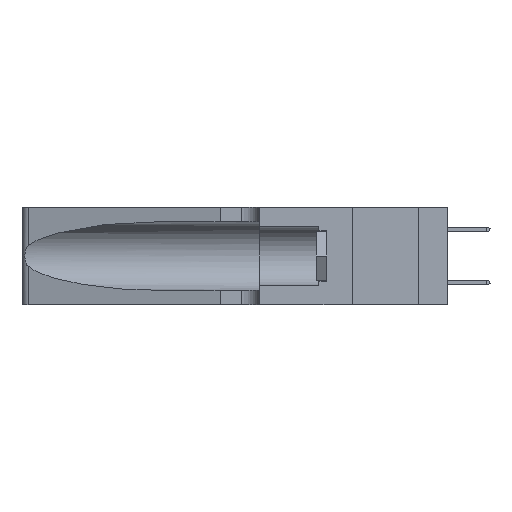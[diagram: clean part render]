
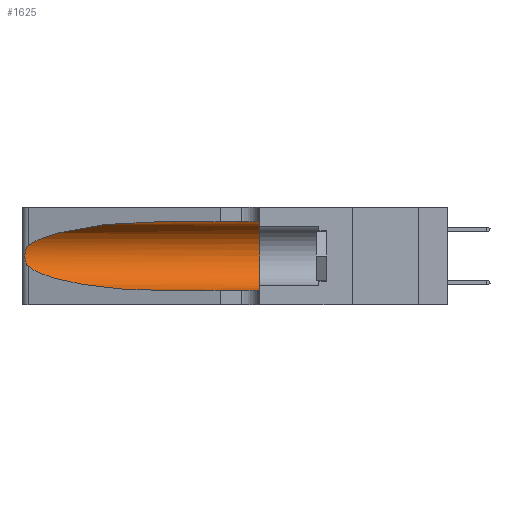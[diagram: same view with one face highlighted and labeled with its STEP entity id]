
A CAD part, left-side view. The second image highlights one B-rep face of the part: STEP entity #1625.
In plain terms, the highlighted cylindrical face has radius 3.308 mm (diameter 6.617 mm), a partial arc.
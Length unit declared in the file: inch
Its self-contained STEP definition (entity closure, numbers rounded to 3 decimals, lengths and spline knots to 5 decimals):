
#87 = VERTEX_POINT ( 'NONE', #21972 ) ;
#1451 = EDGE_CURVE ( 'NONE', #5582, #16488, #2041, .T. ) ;
#1625 = ADVANCED_FACE ( 'NONE', ( #29421 ), #23085, .F. ) ;
#2041 = B_SPLINE_CURVE_WITH_KNOTS ( 'NONE', 3,
 ( #26276, #11181, #11412, #3783, #18534, #28564, #6456, #8677, #25912, #31040, #31164, #11291, #13688, #6216 ),
 .UNSPECIFIED., .F., .F.,
 ( 4, 2, 2, 2, 2, 2, 4 ),
 ( 0., 0.00027, 0.00053, 0.00107, 0.0016, 0.00187, 0.00214 ),
 .UNSPECIFIED. ) ;
#3321 = CARTESIAN_POINT ( 'NONE',  ( 0.1305, 0.35, 0.185 ) ) ;
#3783 = CARTESIAN_POINT ( 'NONE',  ( 0.25787, 1.23484, 0.2124 ) ) ;
#3870 = DIRECTION ( 'NONE',  ( 0., -1., 0. ) ) ;
#4662 = ORIENTED_EDGE ( 'NONE', *, *, #28804, .T. ) ;
#5500 = DIRECTION ( 'NONE',  ( 0., -1., 0. ) ) ;
#5582 = VERTEX_POINT ( 'NONE', #7429 ) ;
#5670 = CARTESIAN_POINT ( 'NONE',  ( 0.25487, 1.22718, 0.14631 ) ) ;
#6216 = CARTESIAN_POINT ( 'NONE',  ( 0.25487, 1.22718, 0.14631 ) ) ;
#6456 = CARTESIAN_POINT ( 'NONE',  ( 0.26075, 1.23896, 0.19203 ) ) ;
#6742 = VERTEX_POINT ( 'NONE', #17976 ) ;
#7429 = CARTESIAN_POINT ( 'NONE',  ( 0.25487, 1.22718, 0.22369 ) ) ;
#7825 = CARTESIAN_POINT ( 'NONE',  ( 0.25487, 1.22718, 0.14631 ) ) ;
#8677 = CARTESIAN_POINT ( 'NONE',  ( 0.26075, 1.23896, 0.178 ) ) ;
#9028 = CARTESIAN_POINT ( 'NONE',  ( 0.18966, 0.96281, 0.05475 ) ) ;
#9557 = ORIENTED_EDGE ( 'NONE', *, *, #1451, .T. ) ;
#9734 = CARTESIAN_POINT ( 'NONE',  ( 0.18966, 0.96281, 0.31525 ) ) ;
#10636 = VERTEX_POINT ( 'NONE', #16142 ) ;
#10696 = DIRECTION ( 'NONE',  ( 0., 1., 0. ) ) ;
#11151 = CARTESIAN_POINT ( 'NONE',  ( 0.1305, 1.61858, 0.05475 ) ) ;
#11181 = CARTESIAN_POINT ( 'NONE',  ( 0.25555, 1.22994, 0.2215 ) ) ;
#11276 = EDGE_CURVE ( 'NONE', #29464, #10636, #20356, .T. ) ;
#11291 = CARTESIAN_POINT ( 'NONE',  ( 0.25639, 1.23186, 0.15144 ) ) ;
#11412 = CARTESIAN_POINT ( 'NONE',  ( 0.25639, 1.23184, 0.21858 ) ) ;
#11788 = ORIENTED_EDGE ( 'NONE', *, *, #14087, .F. ) ;
#13055 = CARTESIAN_POINT ( 'NONE',  ( 0.1305, 1.61858, 0.31525 ) ) ;
#13688 = CARTESIAN_POINT ( 'NONE',  ( 0.25555, 1.22993, 0.14849 ) ) ;
#14087 = EDGE_CURVE ( 'NONE', #10636, #87, #26049, .T. ) ;
#14395 = CARTESIAN_POINT ( 'NONE',  ( 0.2373, 1.15595, 0.28018 ) ) ;
#14895 = ORIENTED_EDGE ( 'NONE', *, *, #11276, .F. ) ;
#15634 = AXIS2_PLACEMENT_3D ( 'NONE', #3321, #10696, #30573 ) ;
#16142 = CARTESIAN_POINT ( 'NONE',  ( 0.1305, 0.35, 0.31525 ) ) ;
#16488 = VERTEX_POINT ( 'NONE', #7825 ) ;
#16965 =( BOUNDED_CURVE ( )  B_SPLINE_CURVE ( 3, ( #17009, #9734, #14395, #19265 ),
 .UNSPECIFIED., .F., .T. ) 
 B_SPLINE_CURVE_WITH_KNOTS ( ( 4, 4 ),
 ( 1.5708, 2.84003 ),
 .UNSPECIFIED. ) 
 CURVE ( )  GEOMETRIC_REPRESENTATION_ITEM ( )  RATIONAL_B_SPLINE_CURVE ( ( 1., 0.87, 0.87, 1. ) ) 
 REPRESENTATION_ITEM ( '' )  );
#17009 = CARTESIAN_POINT ( 'NONE',  ( 0.1305, 0.72297, 0.31525 ) ) ;
#17976 = CARTESIAN_POINT ( 'NONE',  ( 0.1305, 0.72297, 0.05475 ) ) ;
#18033 = VECTOR ( 'NONE', #5500, 39.37008 ) ;
#18534 = CARTESIAN_POINT ( 'NONE',  ( 0.25854, 1.2359, 0.20912 ) ) ;
#18593 = VECTOR ( 'NONE', #3870, 39.37008 ) ;
#19202 = DIRECTION ( 'NONE',  ( 0., 0., -1. ) ) ;
#19265 = CARTESIAN_POINT ( 'NONE',  ( 0.25487, 1.22718, 0.22369 ) ) ;
#19384 = LINE ( 'NONE', #11151, #18593 ) ;
#20272 =( BOUNDED_CURVE ( )  B_SPLINE_CURVE ( 3, ( #5670, #22969, #9028, #26531 ),
 .UNSPECIFIED., .F., .F. ) 
 B_SPLINE_CURVE_WITH_KNOTS ( ( 4, 4 ),
 ( 3.44316, 4.71239 ),
 .UNSPECIFIED. ) 
 CURVE ( )  GEOMETRIC_REPRESENTATION_ITEM ( )  RATIONAL_B_SPLINE_CURVE ( ( 1., 0.87, 0.87, 1. ) ) 
 REPRESENTATION_ITEM ( '' )  );
#20356 = LINE ( 'NONE', #13055, #18033 ) ;
#21972 = CARTESIAN_POINT ( 'NONE',  ( 0.1305, 0.35, 0.05475 ) ) ;
#22969 = CARTESIAN_POINT ( 'NONE',  ( 0.2373, 1.15595, 0.08982 ) ) ;
#23085 = CYLINDRICAL_SURFACE ( 'NONE', #28258, 0.13025 ) ;
#24387 = DIRECTION ( 'NONE',  ( 0., -1., 0. ) ) ;
#24447 = CARTESIAN_POINT ( 'NONE',  ( 0.1305, 0.72297, 0.31525 ) ) ;
#25095 = ORIENTED_EDGE ( 'NONE', *, *, #30487, .T. ) ;
#25207 = ORIENTED_EDGE ( 'NONE', *, *, #27077, .T. ) ;
#25912 = CARTESIAN_POINT ( 'NONE',  ( 0.26017, 1.23833, 0.17102 ) ) ;
#26049 = CIRCLE ( 'NONE', #15634, 0.13025 ) ;
#26276 = CARTESIAN_POINT ( 'NONE',  ( 0.25487, 1.22718, 0.22369 ) ) ;
#26531 = CARTESIAN_POINT ( 'NONE',  ( 0.1305, 0.72297, 0.05475 ) ) ;
#27077 = EDGE_CURVE ( 'NONE', #29464, #5582, #16965, .T. ) ;
#28258 = AXIS2_PLACEMENT_3D ( 'NONE', #31476, #24387, #19202 ) ;
#28564 = CARTESIAN_POINT ( 'NONE',  ( 0.26018, 1.23835, 0.19895 ) ) ;
#28804 = EDGE_CURVE ( 'NONE', #6742, #87, #19384, .T. ) ;
#29421 = FACE_OUTER_BOUND ( 'NONE', #31226, .T. ) ;
#29464 = VERTEX_POINT ( 'NONE', #24447 ) ;
#30487 = EDGE_CURVE ( 'NONE', #16488, #6742, #20272, .T. ) ;
#30573 = DIRECTION ( 'NONE',  ( 0., 0., 1. ) ) ;
#31040 = CARTESIAN_POINT ( 'NONE',  ( 0.25856, 1.23593, 0.16098 ) ) ;
#31164 = CARTESIAN_POINT ( 'NONE',  ( 0.25789, 1.23486, 0.15765 ) ) ;
#31226 = EDGE_LOOP ( 'NONE', ( #25207, #9557, #25095, #4662, #11788, #14895 ) ) ;
#31476 = CARTESIAN_POINT ( 'NONE',  ( 0.1305, 1.61858, 0.185 ) ) ;
